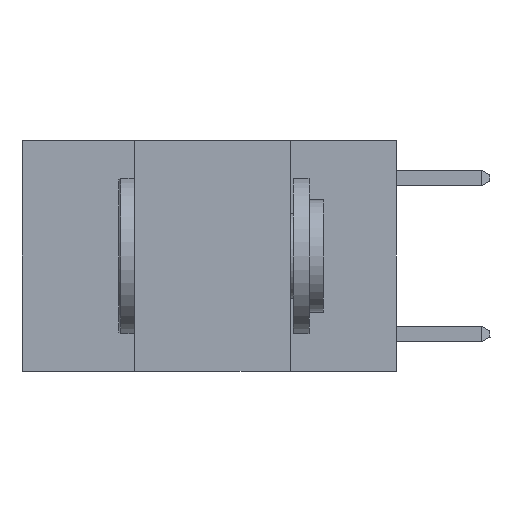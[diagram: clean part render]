
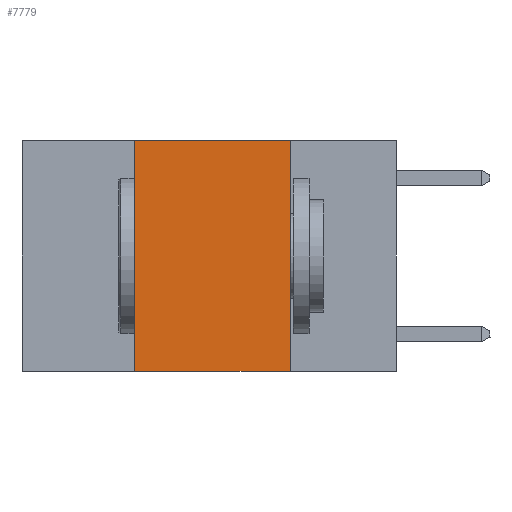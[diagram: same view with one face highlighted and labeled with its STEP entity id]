
A CAD part, left-side view. The second image highlights one B-rep face of the part: STEP entity #7779.
In plain terms, the highlighted planar face has unit normal (-1, 0, 0).
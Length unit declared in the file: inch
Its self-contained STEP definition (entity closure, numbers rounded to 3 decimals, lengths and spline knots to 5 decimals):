
#2119 = PLANE ( 'NONE',  #17136 ) ;
#2437 = LINE ( 'NONE', #17186, #18157 ) ;
#3865 = DIRECTION ( 'NONE',  ( 0., 0., 1. ) ) ;
#4293 = DIRECTION ( 'NONE',  ( 1., 0., 0. ) ) ;
#4327 = CARTESIAN_POINT ( 'NONE',  ( 0., 0.17, 0. ) ) ;
#4464 = CARTESIAN_POINT ( 'NONE',  ( 0., 0.6, -0.37 ) ) ;
#5267 = VECTOR ( 'NONE', #25349, 39.37008 ) ;
#6774 = VERTEX_POINT ( 'NONE', #10210 ) ;
#7166 = CARTESIAN_POINT ( 'NONE',  ( 0., 0.42, 0. ) ) ;
#7476 = VERTEX_POINT ( 'NONE', #7166 ) ;
#7779 = ADVANCED_FACE ( 'NONE', ( #18786 ), #2119, .F. ) ;
#8621 = CARTESIAN_POINT ( 'NONE',  ( 0., 0.6, 0. ) ) ;
#9063 = EDGE_CURVE ( 'NONE', #9766, #7476, #26608, .T. ) ;
#9766 = VERTEX_POINT ( 'NONE', #20805 ) ;
#10210 = CARTESIAN_POINT ( 'NONE',  ( 0., 0.17, -0.37 ) ) ;
#11911 = EDGE_CURVE ( 'NONE', #9766, #6774, #26813, .T. ) ;
#13862 = EDGE_LOOP ( 'NONE', ( #18258, #18365, #19479, #19649 ) ) ;
#14347 = LINE ( 'NONE', #8621, #24701 ) ;
#14490 = CARTESIAN_POINT ( 'NONE',  ( 0., 0.42, 0. ) ) ;
#15457 = EDGE_CURVE ( 'NONE', #19619, #6774, #2437, .T. ) ;
#17098 = CARTESIAN_POINT ( 'NONE',  ( 0., 0.6, 0. ) ) ;
#17136 = AXIS2_PLACEMENT_3D ( 'NONE', #17098, #4293, #19212 ) ;
#17186 = CARTESIAN_POINT ( 'NONE',  ( 0., 0.17, 0. ) ) ;
#18157 = VECTOR ( 'NONE', #23291, 39.37008 ) ;
#18258 = ORIENTED_EDGE ( 'NONE', *, *, #15457, .F. ) ;
#18365 = ORIENTED_EDGE ( 'NONE', *, *, #24301, .F. ) ;
#18786 = FACE_OUTER_BOUND ( 'NONE', #13862, .T. ) ;
#19212 = DIRECTION ( 'NONE',  ( 0., 0., -1. ) ) ;
#19479 = ORIENTED_EDGE ( 'NONE', *, *, #9063, .F. ) ;
#19619 = VERTEX_POINT ( 'NONE', #4327 ) ;
#19649 = ORIENTED_EDGE ( 'NONE', *, *, #11911, .T. ) ;
#20805 = CARTESIAN_POINT ( 'NONE',  ( 0., 0.42, -0.37 ) ) ;
#23282 = DIRECTION ( 'NONE',  ( 0., -1., 0. ) ) ;
#23291 = DIRECTION ( 'NONE',  ( 0., 0., -1. ) ) ;
#24301 = EDGE_CURVE ( 'NONE', #7476, #19619, #14347, .T. ) ;
#24701 = VECTOR ( 'NONE', #23282, 39.37008 ) ;
#25349 = DIRECTION ( 'NONE',  ( 0., -1., 0. ) ) ;
#25958 = VECTOR ( 'NONE', #3865, 39.37008 ) ;
#26608 = LINE ( 'NONE', #14490, #25958 ) ;
#26813 = LINE ( 'NONE', #4464, #5267 ) ;
